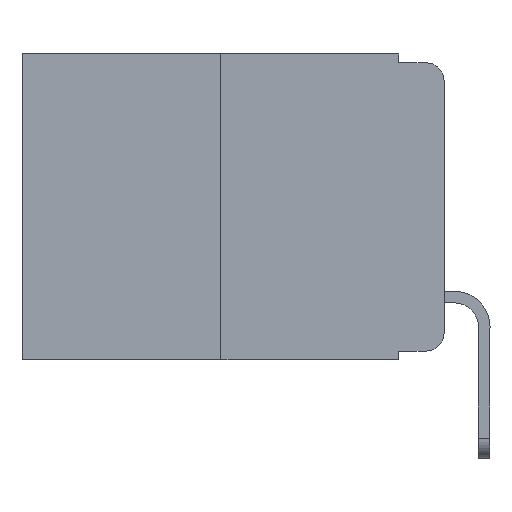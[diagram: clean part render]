
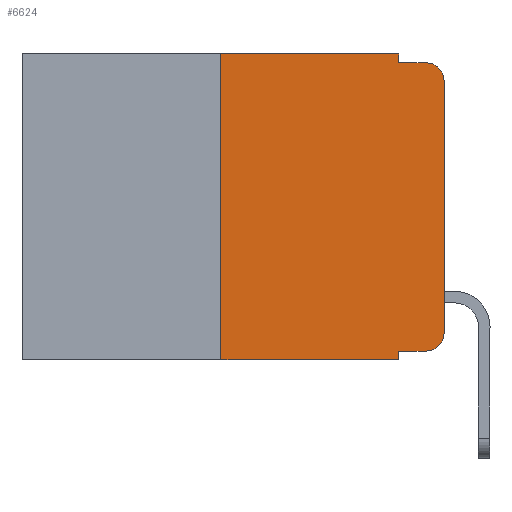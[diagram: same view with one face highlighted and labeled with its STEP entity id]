
A CAD part, left-side view. The second image highlights one B-rep face of the part: STEP entity #6624.
In plain terms, the highlighted planar face has unit normal (-1, 0, 0).
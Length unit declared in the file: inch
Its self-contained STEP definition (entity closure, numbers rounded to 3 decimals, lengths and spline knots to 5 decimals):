
#101 = ORIENTED_EDGE ( 'NONE', *, *, #5477, .F. ) ;
#163 = VECTOR ( 'NONE', #4956, 39.37008 ) ;
#242 = VECTOR ( 'NONE', #902, 39.37008 ) ;
#902 = DIRECTION ( 'NONE',  ( 0., 0., 1. ) ) ;
#987 = ORIENTED_EDGE ( 'NONE', *, *, #5456, .T. ) ;
#1218 = VERTEX_POINT ( 'NONE', #9422 ) ;
#1268 = CARTESIAN_POINT ( 'NONE',  ( 0., 0.25, 0. ) ) ;
#1288 = CARTESIAN_POINT ( 'NONE',  ( 0., 0., -0.313 ) ) ;
#1413 = VERTEX_POINT ( 'NONE', #4897 ) ;
#1674 = ORIENTED_EDGE ( 'NONE', *, *, #6339, .T. ) ;
#1732 = VECTOR ( 'NONE', #5363, 39.37008 ) ;
#2625 = ORIENTED_EDGE ( 'NONE', *, *, #5500, .F. ) ;
#2649 = VECTOR ( 'NONE', #5727, 39.37008 ) ;
#3315 = LINE ( 'NONE', #10091, #163 ) ;
#3409 = DIRECTION ( 'NONE',  ( -1., 0., 0. ) ) ;
#3452 = DIRECTION ( 'NONE',  ( 0., 0., -1. ) ) ;
#3510 = ORIENTED_EDGE ( 'NONE', *, *, #6207, .F. ) ;
#3660 = FACE_OUTER_BOUND ( 'NONE', #5207, .T. ) ;
#4209 = VECTOR ( 'NONE', #5174, 39.37008 ) ;
#4214 = CARTESIAN_POINT ( 'NONE',  ( 0., 0.473, 0. ) ) ;
#4250 = CARTESIAN_POINT ( 'NONE',  ( 0., 0.051, 0. ) ) ;
#4325 = CARTESIAN_POINT ( 'NONE',  ( 0., 0.051, -0.01 ) ) ;
#4576 = CARTESIAN_POINT ( 'NONE',  ( 0., 0.051, -0.01 ) ) ;
#4587 = DIRECTION ( 'NONE',  ( 1., 0., 0. ) ) ;
#4703 = LINE ( 'NONE', #12061, #9907 ) ;
#4776 = CARTESIAN_POINT ( 'NONE',  ( 0., 0.051, -0.333 ) ) ;
#4897 = CARTESIAN_POINT ( 'NONE',  ( 0., 0.02, -0.01 ) ) ;
#4956 = DIRECTION ( 'NONE',  ( 0., 0., 1. ) ) ;
#5174 = DIRECTION ( 'NONE',  ( 0., -1., 0. ) ) ;
#5207 = EDGE_LOOP ( 'NONE', ( #6116, #987, #101, #2625, #7214, #3510, #5529, #7056, #1674, #10297 ) ) ;
#5221 = LINE ( 'NONE', #4214, #1732 ) ;
#5363 = DIRECTION ( 'NONE',  ( 0., -1., 0. ) ) ;
#5370 = LINE ( 'NONE', #11744, #7574 ) ;
#5379 = EDGE_CURVE ( 'NONE', #5596, #9192, #9128, .T. ) ;
#5388 = CARTESIAN_POINT ( 'NONE',  ( 0., 0., -0.03 ) ) ;
#5456 = EDGE_CURVE ( 'NONE', #9192, #1413, #8526, .T. ) ;
#5477 = EDGE_CURVE ( 'NONE', #7363, #1413, #10782, .T. ) ;
#5500 = EDGE_CURVE ( 'NONE', #5871, #7363, #5370, .T. ) ;
#5529 = ORIENTED_EDGE ( 'NONE', *, *, #7745, .T. ) ;
#5557 = VERTEX_POINT ( 'NONE', #4776 ) ;
#5596 = VERTEX_POINT ( 'NONE', #1288 ) ;
#5727 = DIRECTION ( 'NONE',  ( 0., -1., 0. ) ) ;
#5871 = VERTEX_POINT ( 'NONE', #4250 ) ;
#5926 = VERTEX_POINT ( 'NONE', #6648 ) ;
#6116 = ORIENTED_EDGE ( 'NONE', *, *, #5379, .T. ) ;
#6207 = EDGE_CURVE ( 'NONE', #5926, #11408, #3315, .T. ) ;
#6245 = EDGE_CURVE ( 'NONE', #5557, #1218, #8142, .T. ) ;
#6339 = EDGE_CURVE ( 'NONE', #5557, #13117, #12021, .T. ) ;
#6434 = DIRECTION ( 'NONE',  ( -1., 0., 0. ) ) ;
#6624 = ADVANCED_FACE ( 'NONE', ( #3660 ), #10753, .F. ) ;
#6648 = CARTESIAN_POINT ( 'NONE',  ( 0., 0.25, -0.343 ) ) ;
#6759 = CARTESIAN_POINT ( 'NONE',  ( 0., 0.473, 0. ) ) ;
#7056 = ORIENTED_EDGE ( 'NONE', *, *, #6245, .F. ) ;
#7214 = ORIENTED_EDGE ( 'NONE', *, *, #7910, .F. ) ;
#7363 = VERTEX_POINT ( 'NONE', #4325 ) ;
#7386 = CARTESIAN_POINT ( 'NONE',  ( 0., 0.051, -0.333 ) ) ;
#7574 = VECTOR ( 'NONE', #3452, 39.37008 ) ;
#7687 = AXIS2_PLACEMENT_3D ( 'NONE', #6759, #4587, #11709 ) ;
#7719 = AXIS2_PLACEMENT_3D ( 'NONE', #12289, #6434, #13219 ) ;
#7745 = EDGE_CURVE ( 'NONE', #5926, #1218, #4703, .T. ) ;
#7910 = EDGE_CURVE ( 'NONE', #11408, #5871, #5221, .T. ) ;
#8142 = LINE ( 'NONE', #12068, #10403 ) ;
#8526 = CIRCLE ( 'NONE', #8932, 0.02 ) ;
#8932 = AXIS2_PLACEMENT_3D ( 'NONE', #9780, #3409, #10745 ) ;
#9128 = LINE ( 'NONE', #13425, #242 ) ;
#9192 = VERTEX_POINT ( 'NONE', #5388 ) ;
#9422 = CARTESIAN_POINT ( 'NONE',  ( 0., 0.051, -0.343 ) ) ;
#9780 = CARTESIAN_POINT ( 'NONE',  ( 0., 0.02, -0.03 ) ) ;
#9907 = VECTOR ( 'NONE', #12999, 39.37008 ) ;
#10091 = CARTESIAN_POINT ( 'NONE',  ( 0., 0.25, 0. ) ) ;
#10274 = EDGE_CURVE ( 'NONE', #13117, #5596, #10889, .T. ) ;
#10297 = ORIENTED_EDGE ( 'NONE', *, *, #10274, .T. ) ;
#10403 = VECTOR ( 'NONE', #13009, 39.37008 ) ;
#10742 = CARTESIAN_POINT ( 'NONE',  ( 0., 0.02, -0.333 ) ) ;
#10745 = DIRECTION ( 'NONE',  ( 0., 0., -1. ) ) ;
#10753 = PLANE ( 'NONE',  #7687 ) ;
#10782 = LINE ( 'NONE', #4576, #2649 ) ;
#10889 = CIRCLE ( 'NONE', #7719, 0.02 ) ;
#11408 = VERTEX_POINT ( 'NONE', #1268 ) ;
#11709 = DIRECTION ( 'NONE',  ( 0., 0., -1. ) ) ;
#11744 = CARTESIAN_POINT ( 'NONE',  ( 0., 0.051, 0. ) ) ;
#12021 = LINE ( 'NONE', #7386, #4209 ) ;
#12061 = CARTESIAN_POINT ( 'NONE',  ( 0., 0.473, -0.343 ) ) ;
#12068 = CARTESIAN_POINT ( 'NONE',  ( 0., 0.051, 0. ) ) ;
#12289 = CARTESIAN_POINT ( 'NONE',  ( 0., 0.02, -0.313 ) ) ;
#12999 = DIRECTION ( 'NONE',  ( 0., -1., 0. ) ) ;
#13009 = DIRECTION ( 'NONE',  ( 0., 0., -1. ) ) ;
#13117 = VERTEX_POINT ( 'NONE', #10742 ) ;
#13219 = DIRECTION ( 'NONE',  ( 0., 0., -1. ) ) ;
#13425 = CARTESIAN_POINT ( 'NONE',  ( 0., 0., 0. ) ) ;
